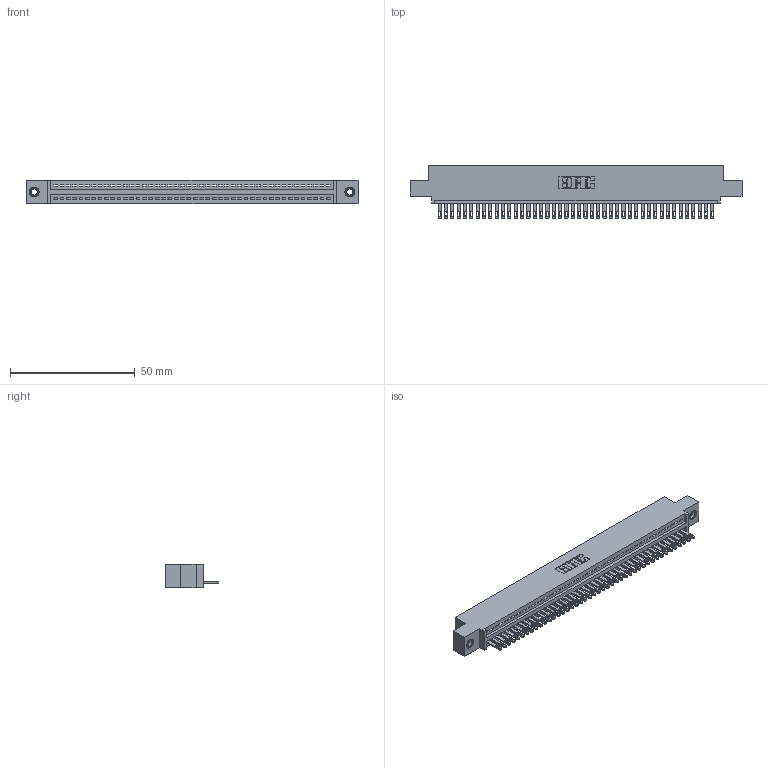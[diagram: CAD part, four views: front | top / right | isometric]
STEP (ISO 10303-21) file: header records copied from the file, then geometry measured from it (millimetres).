
FILE_DESCRIPTION (( 'STEP AP203' ), '1' );
FILE_NAME ('895-044-500-407.STEP', '2020-09-27T02:55:37', ( '' ), ( '' ), 'SwSTEP 2.0', 'SolidWorks 2020', '' );
FILE_SCHEMA (( 'CONFIG_CONTROL_DESIGN' ));
Length unit declared in the file: inch
Products named in the file (4): 845 Part_0.110 Offset - 0.156 Dia-TI; 895-044-500-407; 345-292-001_345-293-100; 345-250-001_345-250-005-103
Assembly tree (47 placements, depth 2):
  895-044-500-407
    845 Part_0.110 Offset - 0.156 Dia-TI
    345-292-001_345-293-100  x44
    345-250-001_345-250-005-103  x2
Bounding box: 132.97 x 21.51 x 9.4 mm (x, y, z)
Volume: 12586.3 mm3; surface area: 16966.4 mm2
Topology: 47 solids, 47 shells, 2566 faces, 7881 edges, 5246 vertices
Faces by surface type: plane 1612, cylinder 938, cone 12, torus 4
Entity records: 34094 total; most frequent: CARTESIAN_POINT 5887, ORIENTED_EDGE 5858, DIRECTION 5167, EDGE_CURVE 2929, LINE 2597, VECTOR 2597, VERTEX_POINT 1948, AXIS2_PLACEMENT_3D 1285
